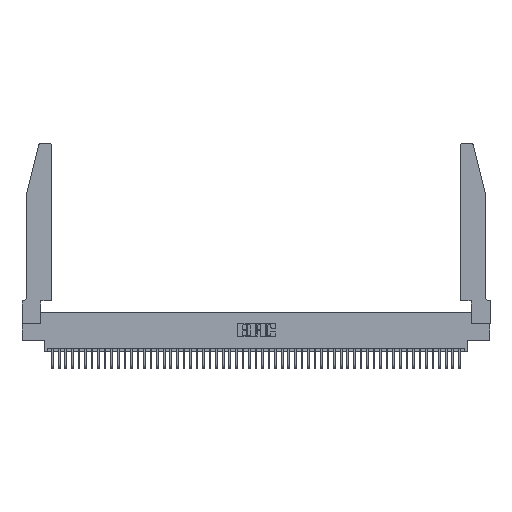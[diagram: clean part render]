
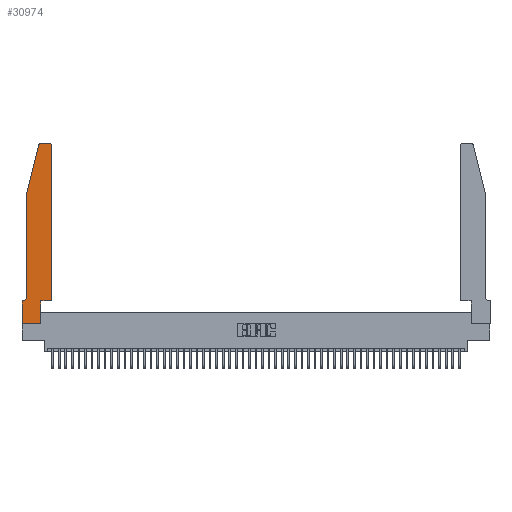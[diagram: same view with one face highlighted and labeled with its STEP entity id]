
A CAD part, top view. The second image highlights one B-rep face of the part: STEP entity #30974.
In plain terms, the highlighted planar face has unit normal (0, 0, 1).
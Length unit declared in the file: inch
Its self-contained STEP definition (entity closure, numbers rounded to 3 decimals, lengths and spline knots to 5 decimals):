
#55 = DIRECTION ( 'NONE',  ( -1., 0., 0. ) ) ;
#344 = CARTESIAN_POINT ( 'NONE',  ( 0., 0.35, 0.37 ) ) ;
#695 = VERTEX_POINT ( 'NONE', #11600 ) ;
#1308 = CARTESIAN_POINT ( 'NONE',  ( 0., 0.35, 0.37 ) ) ;
#1441 = DIRECTION ( 'NONE',  ( 0., -1., 0. ) ) ;
#4282 = EDGE_CURVE ( 'NONE', #22653, #28743, #17413, .T. ) ;
#4535 = DIRECTION ( 'NONE',  ( 0., 0., -1. ) ) ;
#4668 = ORIENTED_EDGE ( 'NONE', *, *, #38603, .T. ) ;
#5513 = CIRCLE ( 'NONE', #13472, 0.03 ) ;
#5541 = DIRECTION ( 'NONE',  ( 1., 0., 0. ) ) ;
#6412 = VECTOR ( 'NONE', #48892, 39.37008 ) ;
#6615 = CIRCLE ( 'NONE', #41916, 0.07 ) ;
#6621 = LINE ( 'NONE', #11983, #16394 ) ;
#7765 = DIRECTION ( 'NONE',  ( 0., 1., 0. ) ) ;
#8358 = AXIS2_PLACEMENT_3D ( 'NONE', #1308, #34272, #9734 ) ;
#9441 = CARTESIAN_POINT ( 'NONE',  ( 0.2605, 2.75, 0.37 ) ) ;
#9734 = DIRECTION ( 'NONE',  ( 1., 0., 0. ) ) ;
#10672 = DIRECTION ( 'NONE',  ( 0., 0., 1. ) ) ;
#10745 = CARTESIAN_POINT ( 'NONE',  ( 0.284, 2.72, 0.37 ) ) ;
#10834 = ORIENTED_EDGE ( 'NONE', *, *, #43460, .T. ) ;
#11322 = EDGE_CURVE ( 'NONE', #26223, #45460, #23058, .T. ) ;
#11600 = CARTESIAN_POINT ( 'NONE',  ( 0.2865, 0.35, 0.37 ) ) ;
#11983 = CARTESIAN_POINT ( 'NONE',  ( 0.2865, 0.35, 0.37 ) ) ;
#12161 = CARTESIAN_POINT ( 'NONE',  ( 0.4505, 0.35, 0.37 ) ) ;
#12742 = EDGE_CURVE ( 'NONE', #52410, #51572, #21629, .T. ) ;
#13472 = AXIS2_PLACEMENT_3D ( 'NONE', #10745, #39347, #14928 ) ;
#13924 = VECTOR ( 'NONE', #5541, 39.37008 ) ;
#14548 = ORIENTED_EDGE ( 'NONE', *, *, #20130, .T. ) ;
#14928 = DIRECTION ( 'NONE',  ( 1., 0., 0. ) ) ;
#15603 = CARTESIAN_POINT ( 'NONE',  ( 0.25487, 2.72718, 0.37 ) ) ;
#16007 = VERTEX_POINT ( 'NONE', #25703 ) ;
#16172 = CARTESIAN_POINT ( 'NONE',  ( 0.0755, 0.35, 0.37 ) ) ;
#16394 = VECTOR ( 'NONE', #7765, 39.37008 ) ;
#16672 = CARTESIAN_POINT ( 'NONE',  ( 0.4205, 2.75, 0.37 ) ) ;
#17413 = LINE ( 'NONE', #9441, #48646 ) ;
#17653 = ORIENTED_EDGE ( 'NONE', *, *, #12742, .T. ) ;
#17962 = VERTEX_POINT ( 'NONE', #344 ) ;
#18581 = ORIENTED_EDGE ( 'NONE', *, *, #32051, .T. ) ;
#19926 = DIRECTION ( 'NONE',  ( 1., 0., 0. ) ) ;
#20130 = EDGE_CURVE ( 'NONE', #45460, #52807, #33305, .T. ) ;
#21629 = LINE ( 'NONE', #23828, #51566 ) ;
#21985 = PLANE ( 'NONE',  #8358 ) ;
#22653 = VERTEX_POINT ( 'NONE', #16672 ) ;
#22858 = CARTESIAN_POINT ( 'NONE',  ( 0., 0., 0.37 ) ) ;
#23058 = LINE ( 'NONE', #38762, #43430 ) ;
#23434 = EDGE_CURVE ( 'NONE', #17962, #52410, #41501, .T. ) ;
#23828 = CARTESIAN_POINT ( 'NONE',  ( 0., 0., 0.37 ) ) ;
#24709 = EDGE_CURVE ( 'NONE', #695, #26233, #46469, .T. ) ;
#25099 = CIRCLE ( 'NONE', #48999, 0.03 ) ;
#25703 = CARTESIAN_POINT ( 'NONE',  ( 0.0055, 0.35, 0.37 ) ) ;
#26223 = VERTEX_POINT ( 'NONE', #15603 ) ;
#26233 = VERTEX_POINT ( 'NONE', #40193 ) ;
#27820 = FACE_OUTER_BOUND ( 'NONE', #40654, .T. ) ;
#28743 = VERTEX_POINT ( 'NONE', #30049 ) ;
#29184 = CARTESIAN_POINT ( 'NONE',  ( 0.0055, 0.42, 0.37 ) ) ;
#29552 = CARTESIAN_POINT ( 'NONE',  ( 0.0755, 0.42, 0.37 ) ) ;
#30049 = CARTESIAN_POINT ( 'NONE',  ( 0.284, 2.75, 0.37 ) ) ;
#30878 = LINE ( 'NONE', #16172, #32182 ) ;
#30974 = ADVANCED_FACE ( 'NONE', ( #27820 ), #21985, .T. ) ;
#32051 = EDGE_CURVE ( 'NONE', #16007, #17962, #30878, .T. ) ;
#32062 = VECTOR ( 'NONE', #32154, 39.37008 ) ;
#32154 = DIRECTION ( 'NONE',  ( 0., -1., 0. ) ) ;
#32182 = VECTOR ( 'NONE', #55, 39.37008 ) ;
#33300 = DIRECTION ( 'NONE',  ( -1., 0., 0. ) ) ;
#33305 = LINE ( 'NONE', #44231, #32062 ) ;
#33532 = CARTESIAN_POINT ( 'NONE',  ( 0.0755, 2., 0.37 ) ) ;
#33978 = DIRECTION ( 'NONE',  ( -1., 0., 0. ) ) ;
#34034 = VERTEX_POINT ( 'NONE', #39093 ) ;
#34272 = DIRECTION ( 'NONE',  ( 0., 0., 1. ) ) ;
#34417 = CARTESIAN_POINT ( 'NONE',  ( 0., 0., 0.37 ) ) ;
#35195 = CARTESIAN_POINT ( 'NONE',  ( 0.4205, 2.72, 0.37 ) ) ;
#35924 = ORIENTED_EDGE ( 'NONE', *, *, #4282, .T. ) ;
#37887 = ORIENTED_EDGE ( 'NONE', *, *, #50225, .T. ) ;
#38270 = ORIENTED_EDGE ( 'NONE', *, *, #24709, .T. ) ;
#38603 = EDGE_CURVE ( 'NONE', #26233, #34034, #39172, .T. ) ;
#38762 = CARTESIAN_POINT ( 'NONE',  ( 0.0755, 2., 0.37 ) ) ;
#38875 = EDGE_CURVE ( 'NONE', #34034, #22653, #25099, .T. ) ;
#39093 = CARTESIAN_POINT ( 'NONE',  ( 0.4505, 2.72, 0.37 ) ) ;
#39172 = LINE ( 'NONE', #12161, #6412 ) ;
#39290 = DIRECTION ( 'NONE',  ( 1., 0., 0. ) ) ;
#39347 = DIRECTION ( 'NONE',  ( 0., 0., 1. ) ) ;
#39586 = ORIENTED_EDGE ( 'NONE', *, *, #52757, .T. ) ;
#40193 = CARTESIAN_POINT ( 'NONE',  ( 0.4505, 0.35, 0.37 ) ) ;
#40654 = EDGE_LOOP ( 'NONE', ( #35924, #37887, #48986, #14548, #39586, #18581, #51363, #17653, #10834, #38270, #4668, #42328 ) ) ;
#41501 = LINE ( 'NONE', #34417, #52362 ) ;
#41761 = CARTESIAN_POINT ( 'NONE',  ( 0.2865, 0., 0.37 ) ) ;
#41916 = AXIS2_PLACEMENT_3D ( 'NONE', #29184, #4535, #33300 ) ;
#42328 = ORIENTED_EDGE ( 'NONE', *, *, #38875, .T. ) ;
#43430 = VECTOR ( 'NONE', #51022, 39.37008 ) ;
#43460 = EDGE_CURVE ( 'NONE', #51572, #695, #6621, .T. ) ;
#44231 = CARTESIAN_POINT ( 'NONE',  ( 0.0755, 2., 0.37 ) ) ;
#45460 = VERTEX_POINT ( 'NONE', #33532 ) ;
#46386 = CARTESIAN_POINT ( 'NONE',  ( 0.4505, 0.35, 0.37 ) ) ;
#46469 = LINE ( 'NONE', #46386, #13924 ) ;
#48646 = VECTOR ( 'NONE', #33978, 39.37008 ) ;
#48892 = DIRECTION ( 'NONE',  ( 0., 1., 0. ) ) ;
#48986 = ORIENTED_EDGE ( 'NONE', *, *, #11322, .T. ) ;
#48999 = AXIS2_PLACEMENT_3D ( 'NONE', #35195, #10672, #39290 ) ;
#50225 = EDGE_CURVE ( 'NONE', #28743, #26223, #5513, .T. ) ;
#51022 = DIRECTION ( 'NONE',  ( -0.239, -0.971, 0. ) ) ;
#51363 = ORIENTED_EDGE ( 'NONE', *, *, #23434, .T. ) ;
#51566 = VECTOR ( 'NONE', #19926, 39.37008 ) ;
#51572 = VERTEX_POINT ( 'NONE', #41761 ) ;
#52362 = VECTOR ( 'NONE', #1441, 39.37008 ) ;
#52410 = VERTEX_POINT ( 'NONE', #22858 ) ;
#52757 = EDGE_CURVE ( 'NONE', #52807, #16007, #6615, .T. ) ;
#52807 = VERTEX_POINT ( 'NONE', #29552 ) ;
